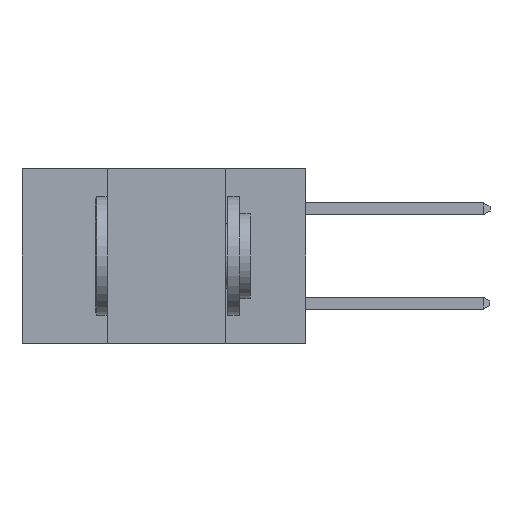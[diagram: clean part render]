
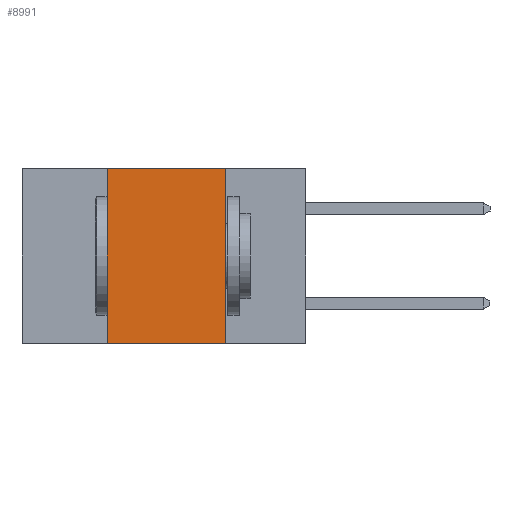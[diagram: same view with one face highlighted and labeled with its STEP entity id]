
A CAD part, left-side view. The second image highlights one B-rep face of the part: STEP entity #8991.
In plain terms, the highlighted planar face has unit normal (-1, 0, 0).
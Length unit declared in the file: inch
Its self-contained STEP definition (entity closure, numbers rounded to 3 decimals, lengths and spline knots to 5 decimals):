
#43 = ORIENTED_EDGE ( 'NONE', *, *, #7035, .F. ) ;
#65 = DIRECTION ( 'NONE',  ( 0., -1., 0. ) ) ;
#119 = CARTESIAN_POINT ( 'NONE',  ( 0., 0.17, 0. ) ) ;
#330 = CARTESIAN_POINT ( 'NONE',  ( 0., 0.42, -0.37 ) ) ;
#494 = DIRECTION ( 'NONE',  ( 0., 0., 1. ) ) ;
#562 = CARTESIAN_POINT ( 'NONE',  ( 0., 0.6, -0.37 ) ) ;
#597 = VERTEX_POINT ( 'NONE', #2044 ) ;
#1112 = ORIENTED_EDGE ( 'NONE', *, *, #3127, .T. ) ;
#1734 = CARTESIAN_POINT ( 'NONE',  ( 0., 0.6, 0. ) ) ;
#2044 = CARTESIAN_POINT ( 'NONE',  ( 0., 0.42, 0. ) ) ;
#2662 = VECTOR ( 'NONE', #3575, 39.37008 ) ;
#2765 = CARTESIAN_POINT ( 'NONE',  ( 0., 0.6, 0. ) ) ;
#2851 = DIRECTION ( 'NONE',  ( 0., 0., -1. ) ) ;
#3127 = EDGE_CURVE ( 'NONE', #5529, #7347, #7795, .T. ) ;
#3575 = DIRECTION ( 'NONE',  ( 0., 0., -1. ) ) ;
#3584 = CARTESIAN_POINT ( 'NONE',  ( 0., 0.17, 0. ) ) ;
#4106 = LINE ( 'NONE', #6668, #6084 ) ;
#5502 = LINE ( 'NONE', #119, #2662 ) ;
#5529 = VERTEX_POINT ( 'NONE', #330 ) ;
#5649 = VECTOR ( 'NONE', #65, 39.37008 ) ;
#5900 = VECTOR ( 'NONE', #6082, 39.37008 ) ;
#6082 = DIRECTION ( 'NONE',  ( 0., -1., 0. ) ) ;
#6084 = VECTOR ( 'NONE', #494, 39.37008 ) ;
#6243 = PLANE ( 'NONE',  #9142 ) ;
#6668 = CARTESIAN_POINT ( 'NONE',  ( 0., 0.42, 0. ) ) ;
#7035 = EDGE_CURVE ( 'NONE', #5529, #597, #4106, .T. ) ;
#7347 = VERTEX_POINT ( 'NONE', #10535 ) ;
#7476 = ORIENTED_EDGE ( 'NONE', *, *, #9902, .F. ) ;
#7795 = LINE ( 'NONE', #562, #5900 ) ;
#7802 = LINE ( 'NONE', #1734, #5649 ) ;
#7865 = DIRECTION ( 'NONE',  ( 1., 0., 0. ) ) ;
#8127 = EDGE_LOOP ( 'NONE', ( #9173, #7476, #43, #1112 ) ) ;
#8991 = ADVANCED_FACE ( 'NONE', ( #9643 ), #6243, .F. ) ;
#9142 = AXIS2_PLACEMENT_3D ( 'NONE', #2765, #7865, #2851 ) ;
#9173 = ORIENTED_EDGE ( 'NONE', *, *, #10595, .F. ) ;
#9643 = FACE_OUTER_BOUND ( 'NONE', #8127, .T. ) ;
#9902 = EDGE_CURVE ( 'NONE', #597, #9982, #7802, .T. ) ;
#9982 = VERTEX_POINT ( 'NONE', #3584 ) ;
#10535 = CARTESIAN_POINT ( 'NONE',  ( 0., 0.17, -0.37 ) ) ;
#10595 = EDGE_CURVE ( 'NONE', #9982, #7347, #5502, .T. ) ;
